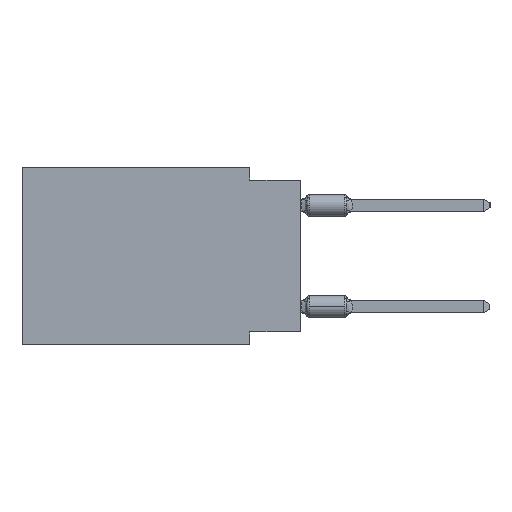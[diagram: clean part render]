
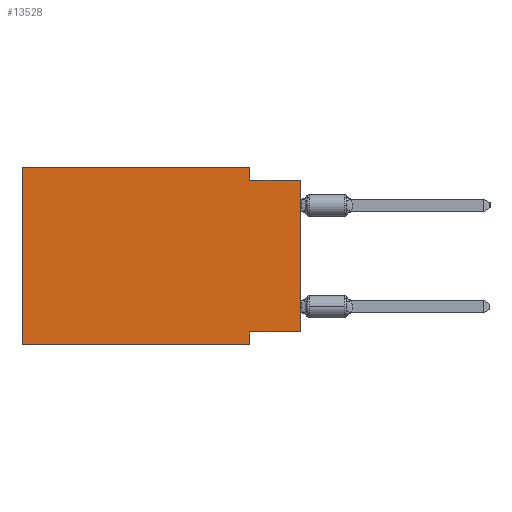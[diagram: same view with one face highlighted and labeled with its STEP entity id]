
A CAD part, left-side view. The second image highlights one B-rep face of the part: STEP entity #13528.
In plain terms, the highlighted planar face has unit normal (-1, 0, 0).
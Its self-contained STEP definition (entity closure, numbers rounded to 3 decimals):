
#14 = CARTESIAN_POINT ( 'NONE',  ( 0., 0., -8.255 ) ) ;
#561 = DIRECTION ( 'NONE',  ( 0., -1., 0. ) ) ;
#3598 = EDGE_LOOP ( 'NONE', ( #39447, #36048, #33827, #12848, #36288, #14740, #9052, #33960 ) ) ;
#5077 = CARTESIAN_POINT ( 'NONE',  ( 0., 0., 0. ) ) ;
#5152 = VECTOR ( 'NONE', #15660, 1000. ) ;
#5610 = LINE ( 'NONE', #39716, #19291 ) ;
#5871 = CARTESIAN_POINT ( 'NONE',  ( 0., 0., -0.635 ) ) ;
#6450 = EDGE_CURVE ( 'NONE', #46798, #29804, #44872, .T. ) ;
#8343 = EDGE_CURVE ( 'NONE', #43466, #46798, #44574, .T. ) ;
#9052 = ORIENTED_EDGE ( 'NONE', *, *, #23124, .F. ) ;
#9831 = EDGE_CURVE ( 'NONE', #42402, #47900, #15404, .T. ) ;
#11949 = EDGE_CURVE ( 'NONE', #41739, #12139, #38457, .T. ) ;
#12139 = VERTEX_POINT ( 'NONE', #5871 ) ;
#12848 = ORIENTED_EDGE ( 'NONE', *, *, #6450, .F. ) ;
#12998 = VECTOR ( 'NONE', #15147, 1000. ) ;
#13014 = DIRECTION ( 'NONE',  ( 0., -1., 0. ) ) ;
#13227 = CARTESIAN_POINT ( 'NONE',  ( 0., 2.54, -8.89 ) ) ;
#13472 = DIRECTION ( 'NONE',  ( 1., 0., 0. ) ) ;
#13528 = ADVANCED_FACE ( 'NONE', ( #43547 ), #32671, .F. ) ;
#14225 = CARTESIAN_POINT ( 'NONE',  ( 0., 2.54, 0. ) ) ;
#14740 = ORIENTED_EDGE ( 'NONE', *, *, #29790, .T. ) ;
#15147 = DIRECTION ( 'NONE',  ( 0., 0., -1. ) ) ;
#15404 = LINE ( 'NONE', #14, #5152 ) ;
#15540 = EDGE_CURVE ( 'NONE', #29804, #41739, #49744, .T. ) ;
#15660 = DIRECTION ( 'NONE',  ( 0., 1., 0. ) ) ;
#16187 = DIRECTION ( 'NONE',  ( 0., 0., 1. ) ) ;
#17046 = VECTOR ( 'NONE', #37790, 1000. ) ;
#17139 = CARTESIAN_POINT ( 'NONE',  ( 0., 2.54, -8.255 ) ) ;
#18174 = VERTEX_POINT ( 'NONE', #13227 ) ;
#18222 = VECTOR ( 'NONE', #13014, 1000. ) ;
#19271 = CARTESIAN_POINT ( 'NONE',  ( 0., 0., -0.635 ) ) ;
#19291 = VECTOR ( 'NONE', #21007, 1000. ) ;
#19625 = VECTOR ( 'NONE', #561, 1000. ) ;
#20086 = LINE ( 'NONE', #20575, #18222 ) ;
#20575 = CARTESIAN_POINT ( 'NONE',  ( 0., 13.97, -8.89 ) ) ;
#20703 = LINE ( 'NONE', #5077, #32885 ) ;
#21007 = DIRECTION ( 'NONE',  ( 0., 0., -1. ) ) ;
#22383 = CARTESIAN_POINT ( 'NONE',  ( 0., 13.97, 0. ) ) ;
#23124 = EDGE_CURVE ( 'NONE', #47900, #18174, #5610, .T. ) ;
#25370 = DIRECTION ( 'NONE',  ( 0., 0., -1. ) ) ;
#27431 = CARTESIAN_POINT ( 'NONE',  ( 0., 2.54, -0.635 ) ) ;
#29137 = CARTESIAN_POINT ( 'NONE',  ( 0., 13.97, 0. ) ) ;
#29790 = EDGE_CURVE ( 'NONE', #43466, #18174, #20086, .T. ) ;
#29804 = VERTEX_POINT ( 'NONE', #43821 ) ;
#31709 = VECTOR ( 'NONE', #40278, 1000. ) ;
#32671 = PLANE ( 'NONE',  #37202 ) ;
#32885 = VECTOR ( 'NONE', #16187, 1000. ) ;
#33827 = ORIENTED_EDGE ( 'NONE', *, *, #15540, .F. ) ;
#33960 = ORIENTED_EDGE ( 'NONE', *, *, #9831, .F. ) ;
#36048 = ORIENTED_EDGE ( 'NONE', *, *, #11949, .F. ) ;
#36237 = CARTESIAN_POINT ( 'NONE',  ( 0., 13.97, -8.89 ) ) ;
#36288 = ORIENTED_EDGE ( 'NONE', *, *, #8343, .F. ) ;
#37202 = AXIS2_PLACEMENT_3D ( 'NONE', #29137, #13472, #25370 ) ;
#37790 = DIRECTION ( 'NONE',  ( 0., -1., 0. ) ) ;
#38457 = LINE ( 'NONE', #19271, #19625 ) ;
#39447 = ORIENTED_EDGE ( 'NONE', *, *, #44217, .T. ) ;
#39716 = CARTESIAN_POINT ( 'NONE',  ( 0., 2.54, -8.89 ) ) ;
#40278 = DIRECTION ( 'NONE',  ( 0., 0., 1. ) ) ;
#41739 = VERTEX_POINT ( 'NONE', #27431 ) ;
#42227 = CARTESIAN_POINT ( 'NONE',  ( 0., 0., -8.255 ) ) ;
#42402 = VERTEX_POINT ( 'NONE', #42227 ) ;
#43466 = VERTEX_POINT ( 'NONE', #36237 ) ;
#43547 = FACE_OUTER_BOUND ( 'NONE', #3598, .T. ) ;
#43821 = CARTESIAN_POINT ( 'NONE',  ( 0., 2.54, 0. ) ) ;
#44217 = EDGE_CURVE ( 'NONE', #42402, #12139, #20703, .T. ) ;
#44574 = LINE ( 'NONE', #47333, #31709 ) ;
#44872 = LINE ( 'NONE', #22383, #17046 ) ;
#46798 = VERTEX_POINT ( 'NONE', #49254 ) ;
#47333 = CARTESIAN_POINT ( 'NONE',  ( 0., 13.97, 0. ) ) ;
#47900 = VERTEX_POINT ( 'NONE', #17139 ) ;
#49254 = CARTESIAN_POINT ( 'NONE',  ( 0., 13.97, 0. ) ) ;
#49744 = LINE ( 'NONE', #14225, #12998 ) ;
